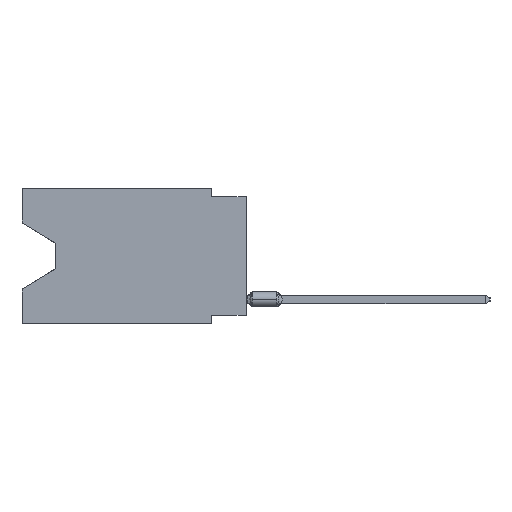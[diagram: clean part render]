
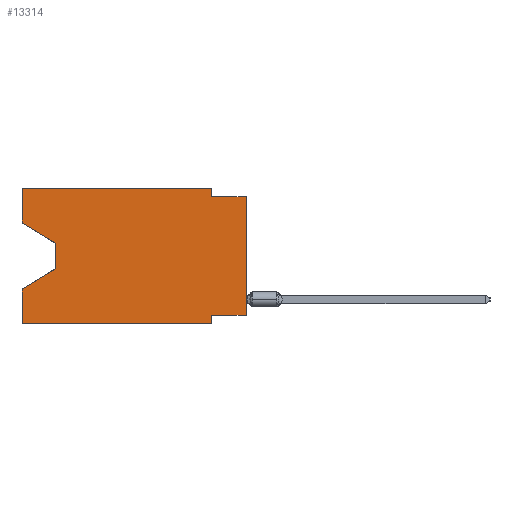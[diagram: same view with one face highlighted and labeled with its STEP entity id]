
A CAD part, left-side view. The second image highlights one B-rep face of the part: STEP entity #13314.
In plain terms, the highlighted planar face has unit normal (-1, 0, 0).
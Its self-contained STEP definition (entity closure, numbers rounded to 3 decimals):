
#986 = VERTEX_POINT ( 'NONE', #59327 ) ;
#2186 = CARTESIAN_POINT ( 'NONE',  ( 0., 2.54, -0.635 ) ) ;
#2293 = ORIENTED_EDGE ( 'NONE', *, *, #56952, .T. ) ;
#3328 = CARTESIAN_POINT ( 'NONE',  ( 0., 0., 0. ) ) ;
#3951 = ORIENTED_EDGE ( 'NONE', *, *, #33238, .F. ) ;
#5158 = ORIENTED_EDGE ( 'NONE', *, *, #75227, .T. ) ;
#5197 = VECTOR ( 'NONE', #63520, 1000. ) ;
#5880 = LINE ( 'NONE', #32619, #67898 ) ;
#6680 = EDGE_LOOP ( 'NONE', ( #49325, #5158, #22884, #3951, #2293, #29119, #49487, #59161, #55448, #43214, #63423, #87908 ) ) ;
#6978 = CARTESIAN_POINT ( 'NONE',  ( 0., 13.97, -5.893 ) ) ;
#7492 = LINE ( 'NONE', #80152, #35210 ) ;
#8286 = LINE ( 'NONE', #44330, #5197 ) ;
#9499 = VERTEX_POINT ( 'NONE', #78850 ) ;
#10076 = EDGE_CURVE ( 'NONE', #77472, #64660, #49139, .T. ) ;
#10237 = EDGE_CURVE ( 'NONE', #66952, #77472, #5880, .T. ) ;
#11423 = VECTOR ( 'NONE', #59196, 1000. ) ;
#11655 = CARTESIAN_POINT ( 'NONE',  ( 0., 16.383, 0. ) ) ;
#13314 = ADVANCED_FACE ( 'NONE', ( #25015 ), #37967, .F. ) ;
#16366 = CARTESIAN_POINT ( 'NONE',  ( 0., 13.97, -4.013 ) ) ;
#18391 = CARTESIAN_POINT ( 'NONE',  ( 0., 16.383, 0. ) ) ;
#20415 = CARTESIAN_POINT ( 'NONE',  ( 0., 0., -9.271 ) ) ;
#20847 = DIRECTION ( 'NONE',  ( 0., 0., -1. ) ) ;
#21541 = CARTESIAN_POINT ( 'NONE',  ( 0., 2.54, 0. ) ) ;
#22052 = LINE ( 'NONE', #3328, #87839 ) ;
#22124 = EDGE_CURVE ( 'NONE', #64660, #84152, #7492, .T. ) ;
#22884 = ORIENTED_EDGE ( 'NONE', *, *, #45092, .T. ) ;
#23010 = DIRECTION ( 'NONE',  ( 0., 1., 0. ) ) ;
#23355 = DIRECTION ( 'NONE',  ( 0., 0., -1. ) ) ;
#24071 = VERTEX_POINT ( 'NONE', #26423 ) ;
#25015 = FACE_OUTER_BOUND ( 'NONE', #6680, .T. ) ;
#25215 = CARTESIAN_POINT ( 'NONE',  ( 0., 2.54, -9.271 ) ) ;
#26423 = CARTESIAN_POINT ( 'NONE',  ( 0., 0., -0.635 ) ) ;
#27993 = VECTOR ( 'NONE', #23355, 1000. ) ;
#28185 = CARTESIAN_POINT ( 'NONE',  ( 0., 16.383, -9.906 ) ) ;
#29119 = ORIENTED_EDGE ( 'NONE', *, *, #73238, .F. ) ;
#30055 = CARTESIAN_POINT ( 'NONE',  ( 0., 13.97, -4.013 ) ) ;
#32172 = DIRECTION ( 'NONE',  ( 0., 0., 1. ) ) ;
#32619 = CARTESIAN_POINT ( 'NONE',  ( 0., 16.383, 0. ) ) ;
#33238 = EDGE_CURVE ( 'NONE', #68258, #67971, #56984, .T. ) ;
#33724 = DIRECTION ( 'NONE',  ( 0., 0.855, -0.519 ) ) ;
#33766 = EDGE_CURVE ( 'NONE', #44711, #36140, #57771, .T. ) ;
#35210 = VECTOR ( 'NONE', #20847, 1000. ) ;
#35637 = EDGE_CURVE ( 'NONE', #66952, #50937, #65877, .T. ) ;
#36140 = VERTEX_POINT ( 'NONE', #25215 ) ;
#36424 = CARTESIAN_POINT ( 'NONE',  ( 0., 0., -9.271 ) ) ;
#37654 = VECTOR ( 'NONE', #64995, 1000. ) ;
#37820 = DIRECTION ( 'NONE',  ( 0., -0.855, -0.519 ) ) ;
#37967 = PLANE ( 'NONE',  #44011 ) ;
#43214 = ORIENTED_EDGE ( 'NONE', *, *, #22124, .F. ) ;
#43419 = LINE ( 'NONE', #30055, #27993 ) ;
#43869 = DIRECTION ( 'NONE',  ( 0., 0., 1. ) ) ;
#44011 = AXIS2_PLACEMENT_3D ( 'NONE', #11655, #58872, #78082 ) ;
#44330 = CARTESIAN_POINT ( 'NONE',  ( 0., 0., -0.635 ) ) ;
#44711 = VERTEX_POINT ( 'NONE', #20415 ) ;
#44790 = VECTOR ( 'NONE', #80860, 1000. ) ;
#45092 = EDGE_CURVE ( 'NONE', #986, #67971, #55075, .T. ) ;
#45393 = CARTESIAN_POINT ( 'NONE',  ( 0., 16.383, -9.906 ) ) ;
#45826 = LINE ( 'NONE', #45393, #11423 ) ;
#46194 = CARTESIAN_POINT ( 'NONE',  ( 0., 16.383, 0. ) ) ;
#49139 = LINE ( 'NONE', #46194, #77812 ) ;
#49325 = ORIENTED_EDGE ( 'NONE', *, *, #35637, .T. ) ;
#49487 = ORIENTED_EDGE ( 'NONE', *, *, #33766, .F. ) ;
#50937 = VERTEX_POINT ( 'NONE', #16366 ) ;
#51241 = EDGE_CURVE ( 'NONE', #84152, #24071, #8286, .T. ) ;
#54111 = EDGE_CURVE ( 'NONE', #44711, #24071, #22052, .T. ) ;
#54794 = VECTOR ( 'NONE', #23010, 1000. ) ;
#54867 = VECTOR ( 'NONE', #37820, 1000. ) ;
#55075 = LINE ( 'NONE', #6978, #72730 ) ;
#55448 = ORIENTED_EDGE ( 'NONE', *, *, #51241, .F. ) ;
#56952 = EDGE_CURVE ( 'NONE', #68258, #9499, #45826, .T. ) ;
#56984 = LINE ( 'NONE', #85070, #37654 ) ;
#57771 = LINE ( 'NONE', #36424, #54794 ) ;
#58872 = DIRECTION ( 'NONE',  ( 1., 0., 0. ) ) ;
#59161 = ORIENTED_EDGE ( 'NONE', *, *, #54111, .T. ) ;
#59196 = DIRECTION ( 'NONE',  ( 0., -1., 0. ) ) ;
#59327 = CARTESIAN_POINT ( 'NONE',  ( 0., 13.97, -5.893 ) ) ;
#59895 = CARTESIAN_POINT ( 'NONE',  ( 0., 2.54, -9.906 ) ) ;
#63423 = ORIENTED_EDGE ( 'NONE', *, *, #10076, .F. ) ;
#63520 = DIRECTION ( 'NONE',  ( 0., -1., 0. ) ) ;
#64660 = VERTEX_POINT ( 'NONE', #21541 ) ;
#64995 = DIRECTION ( 'NONE',  ( 0., 0., 1. ) ) ;
#65877 = LINE ( 'NONE', #73010, #54867 ) ;
#66952 = VERTEX_POINT ( 'NONE', #84303 ) ;
#67898 = VECTOR ( 'NONE', #32172, 1000. ) ;
#67971 = VERTEX_POINT ( 'NONE', #72354 ) ;
#68258 = VERTEX_POINT ( 'NONE', #28185 ) ;
#72354 = CARTESIAN_POINT ( 'NONE',  ( 0., 16.383, -7.36 ) ) ;
#72730 = VECTOR ( 'NONE', #33724, 1000. ) ;
#73010 = CARTESIAN_POINT ( 'NONE',  ( 0., 16.383, -2.546 ) ) ;
#73238 = EDGE_CURVE ( 'NONE', #36140, #9499, #74167, .T. ) ;
#73392 = DIRECTION ( 'NONE',  ( 0., -1., 0. ) ) ;
#74167 = LINE ( 'NONE', #59895, #44790 ) ;
#75227 = EDGE_CURVE ( 'NONE', #50937, #986, #43419, .T. ) ;
#77472 = VERTEX_POINT ( 'NONE', #18391 ) ;
#77812 = VECTOR ( 'NONE', #73392, 1000. ) ;
#78082 = DIRECTION ( 'NONE',  ( 0., 0., -1. ) ) ;
#78850 = CARTESIAN_POINT ( 'NONE',  ( 0., 2.54, -9.906 ) ) ;
#80152 = CARTESIAN_POINT ( 'NONE',  ( 0., 2.54, 0. ) ) ;
#80860 = DIRECTION ( 'NONE',  ( 0., 0., -1. ) ) ;
#84152 = VERTEX_POINT ( 'NONE', #2186 ) ;
#84303 = CARTESIAN_POINT ( 'NONE',  ( 0., 16.383, -2.546 ) ) ;
#85070 = CARTESIAN_POINT ( 'NONE',  ( 0., 16.383, 0. ) ) ;
#87839 = VECTOR ( 'NONE', #43869, 1000. ) ;
#87908 = ORIENTED_EDGE ( 'NONE', *, *, #10237, .F. ) ;
